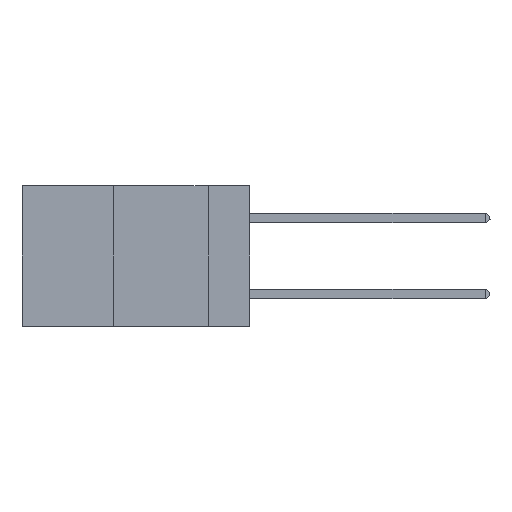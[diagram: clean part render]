
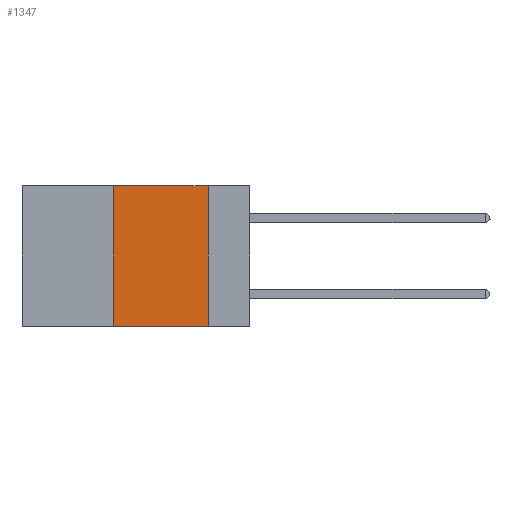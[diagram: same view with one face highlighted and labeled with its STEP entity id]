
A CAD part, left-side view. The second image highlights one B-rep face of the part: STEP entity #1347.
In plain terms, the highlighted planar face has unit normal (-1, 0, 0).
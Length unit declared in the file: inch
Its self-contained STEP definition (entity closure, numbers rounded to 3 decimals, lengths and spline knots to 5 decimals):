
#325 = DIRECTION ( 'NONE',  ( 0., 0., -1. ) ) ;
#943 = ORIENTED_EDGE ( 'NONE', *, *, #19750, .T. ) ;
#1223 = FACE_OUTER_BOUND ( 'NONE', #13552, .T. ) ;
#1347 = ADVANCED_FACE ( 'NONE', ( #1223 ), #10599, .F. ) ;
#1434 = CARTESIAN_POINT ( 'NONE',  ( 0., 0.11, 0. ) ) ;
#1871 = CARTESIAN_POINT ( 'NONE',  ( 0., 0.36, -0.37 ) ) ;
#3138 = VERTEX_POINT ( 'NONE', #18282 ) ;
#3291 = LINE ( 'NONE', #16042, #22684 ) ;
#3518 = DIRECTION ( 'NONE',  ( 0., -1., 0. ) ) ;
#5512 = DIRECTION ( 'NONE',  ( 0., 0., 1. ) ) ;
#5763 = LINE ( 'NONE', #20057, #19952 ) ;
#6823 = EDGE_CURVE ( 'NONE', #3138, #11099, #13930, .T. ) ;
#6938 = CARTESIAN_POINT ( 'NONE',  ( 0., 0.6, 0. ) ) ;
#7015 = DIRECTION ( 'NONE',  ( 0., -1., 0. ) ) ;
#8147 = EDGE_CURVE ( 'NONE', #11099, #14254, #19677, .T. ) ;
#9755 = VERTEX_POINT ( 'NONE', #1871 ) ;
#10246 = DIRECTION ( 'NONE',  ( 0., 0., -1. ) ) ;
#10599 = PLANE ( 'NONE',  #12926 ) ;
#10918 = ORIENTED_EDGE ( 'NONE', *, *, #15687, .F. ) ;
#11099 = VERTEX_POINT ( 'NONE', #1434 ) ;
#11617 = VECTOR ( 'NONE', #7015, 39.37008 ) ;
#12926 = AXIS2_PLACEMENT_3D ( 'NONE', #6938, #22668, #10246 ) ;
#13552 = EDGE_LOOP ( 'NONE', ( #23124, #17581, #10918, #943 ) ) ;
#13930 = LINE ( 'NONE', #19209, #11617 ) ;
#14254 = VERTEX_POINT ( 'NONE', #21665 ) ;
#15406 = VECTOR ( 'NONE', #325, 39.37008 ) ;
#15687 = EDGE_CURVE ( 'NONE', #9755, #3138, #5763, .T. ) ;
#16042 = CARTESIAN_POINT ( 'NONE',  ( 0., 0.6, -0.37 ) ) ;
#17581 = ORIENTED_EDGE ( 'NONE', *, *, #6823, .F. ) ;
#18282 = CARTESIAN_POINT ( 'NONE',  ( 0., 0.36, 0. ) ) ;
#19209 = CARTESIAN_POINT ( 'NONE',  ( 0., 0.6, 0. ) ) ;
#19677 = LINE ( 'NONE', #22850, #15406 ) ;
#19750 = EDGE_CURVE ( 'NONE', #9755, #14254, #3291, .T. ) ;
#19952 = VECTOR ( 'NONE', #5512, 39.37008 ) ;
#20057 = CARTESIAN_POINT ( 'NONE',  ( 0., 0.36, 0. ) ) ;
#21665 = CARTESIAN_POINT ( 'NONE',  ( 0., 0.11, -0.37 ) ) ;
#22668 = DIRECTION ( 'NONE',  ( 1., 0., 0. ) ) ;
#22684 = VECTOR ( 'NONE', #3518, 39.37008 ) ;
#22850 = CARTESIAN_POINT ( 'NONE',  ( 0., 0.11, 0. ) ) ;
#23124 = ORIENTED_EDGE ( 'NONE', *, *, #8147, .F. ) ;
